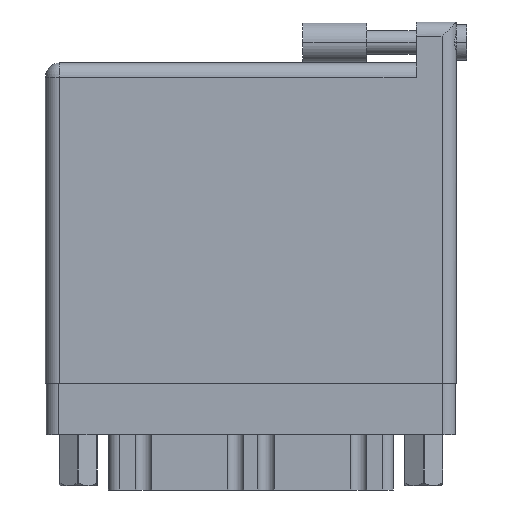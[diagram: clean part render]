
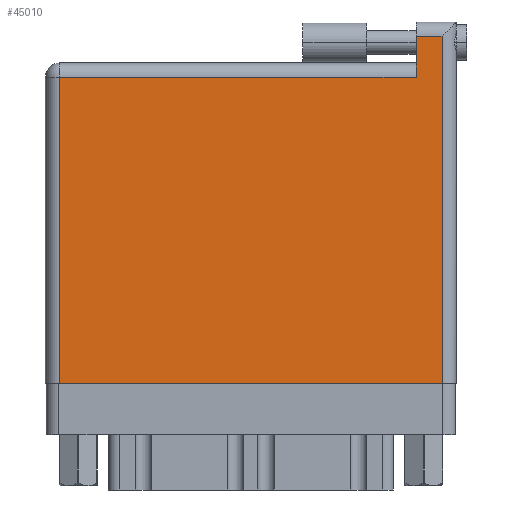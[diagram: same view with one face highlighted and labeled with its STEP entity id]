
A CAD part, front view. The second image highlights one B-rep face of the part: STEP entity #45010.
In plain terms, the highlighted face is planar.
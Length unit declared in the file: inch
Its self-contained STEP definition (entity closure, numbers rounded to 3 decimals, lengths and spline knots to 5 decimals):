
#2031 = ORIENTED_EDGE ( 'NONE', *, *, #35931, .T. ) ;
#2871 = ORIENTED_EDGE ( 'NONE', *, *, #31873, .T. ) ;
#3201 = EDGE_CURVE ( 'NONE', #39734, #8651, #9548, .T. ) ;
#4347 = LINE ( 'NONE', #22516, #9515 ) ;
#5173 = LINE ( 'NONE', #30759, #6973 ) ;
#6319 = CARTESIAN_POINT ( 'NONE',  ( 0.07, 1.496, 0. ) ) ;
#6434 = CARTESIAN_POINT ( 'NONE',  ( 0.07, 0., 0. ) ) ;
#6973 = VECTOR ( 'NONE', #27181, 39.37008 ) ;
#8651 = VERTEX_POINT ( 'NONE', #28313 ) ;
#8986 = PLANE ( 'NONE',  #23909 ) ;
#9228 = CARTESIAN_POINT ( 'NONE',  ( 0., 1.566, 0. ) ) ;
#9515 = VECTOR ( 'NONE', #22991, 39.37008 ) ;
#9548 = LINE ( 'NONE', #6434, #35191 ) ;
#10275 = ORIENTED_EDGE ( 'NONE', *, *, #37749, .T. ) ;
#10689 = LINE ( 'NONE', #10919, #29705 ) ;
#10919 = CARTESIAN_POINT ( 'NONE',  ( 0., 0., 0. ) ) ;
#13112 = DIRECTION ( 'NONE',  ( 0., -1., 0. ) ) ;
#13282 = VECTOR ( 'NONE', #24707, 39.37008 ) ;
#17635 = CARTESIAN_POINT ( 'NONE',  ( 1.938, 1.766, 0. ) ) ;
#18356 = CARTESIAN_POINT ( 'NONE',  ( 1.938, 0., 0. ) ) ;
#19171 = CARTESIAN_POINT ( 'NONE',  ( 1.811, 1.696, 0. ) ) ;
#19236 = EDGE_LOOP ( 'NONE', ( #10275, #20440, #2031, #2871, #24949, #26028 ) ) ;
#20169 = VERTEX_POINT ( 'NONE', #38836 ) ;
#20440 = ORIENTED_EDGE ( 'NONE', *, *, #37817, .T. ) ;
#20455 = DIRECTION ( 'NONE',  ( -1., 0., 0. ) ) ;
#22516 = CARTESIAN_POINT ( 'NONE',  ( 0., 1.496, 0. ) ) ;
#22991 = DIRECTION ( 'NONE',  ( -1., 0., 0. ) ) ;
#23803 = DIRECTION ( 'NONE',  ( 0., 0., -1. ) ) ;
#23909 = AXIS2_PLACEMENT_3D ( 'NONE', #9228, #23803, #20455 ) ;
#24707 = DIRECTION ( 'NONE',  ( -1., 0., 0. ) ) ;
#24949 = ORIENTED_EDGE ( 'NONE', *, *, #36014, .T. ) ;
#25521 = DIRECTION ( 'NONE',  ( 1., 0., 0. ) ) ;
#26028 = ORIENTED_EDGE ( 'NONE', *, *, #3201, .T. ) ;
#26486 = VERTEX_POINT ( 'NONE', #19171 ) ;
#27181 = DIRECTION ( 'NONE',  ( 0., -1., 0. ) ) ;
#28313 = CARTESIAN_POINT ( 'NONE',  ( 0.07, 0., 0. ) ) ;
#29236 = LINE ( 'NONE', #36185, #13282 ) ;
#29705 = VECTOR ( 'NONE', #25521, 39.37008 ) ;
#30759 = CARTESIAN_POINT ( 'NONE',  ( 1.811, 1.766, 0. ) ) ;
#31873 = EDGE_CURVE ( 'NONE', #26486, #45491, #5173, .T. ) ;
#34987 = CARTESIAN_POINT ( 'NONE',  ( 1.811, 1.496, 0. ) ) ;
#35191 = VECTOR ( 'NONE', #13112, 39.37008 ) ;
#35931 = EDGE_CURVE ( 'NONE', #20169, #26486, #29236, .T. ) ;
#36014 = EDGE_CURVE ( 'NONE', #45491, #39734, #4347, .T. ) ;
#36053 = LINE ( 'NONE', #17635, #42706 ) ;
#36185 = CARTESIAN_POINT ( 'NONE',  ( 0., 1.696, 0. ) ) ;
#37749 = EDGE_CURVE ( 'NONE', #8651, #39568, #10689, .T. ) ;
#37817 = EDGE_CURVE ( 'NONE', #39568, #20169, #36053, .T. ) ;
#38637 = FACE_OUTER_BOUND ( 'NONE', #19236, .T. ) ;
#38836 = CARTESIAN_POINT ( 'NONE',  ( 1.938, 1.696, 0. ) ) ;
#39568 = VERTEX_POINT ( 'NONE', #18356 ) ;
#39734 = VERTEX_POINT ( 'NONE', #6319 ) ;
#42706 = VECTOR ( 'NONE', #43678, 39.37008 ) ;
#43678 = DIRECTION ( 'NONE',  ( 0., 1., 0. ) ) ;
#45010 = ADVANCED_FACE ( 'NONE', ( #38637 ), #8986, .F. ) ;
#45491 = VERTEX_POINT ( 'NONE', #34987 ) ;
